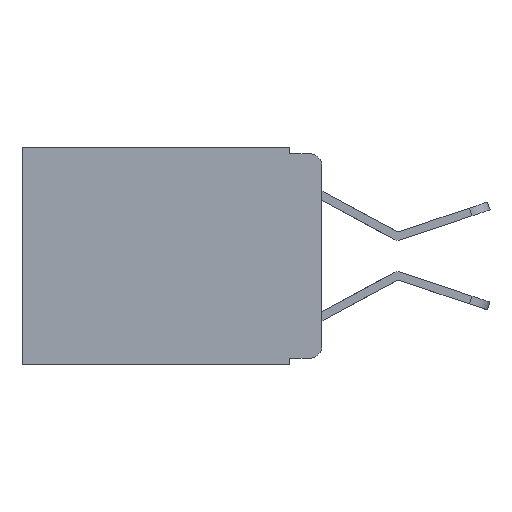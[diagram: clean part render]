
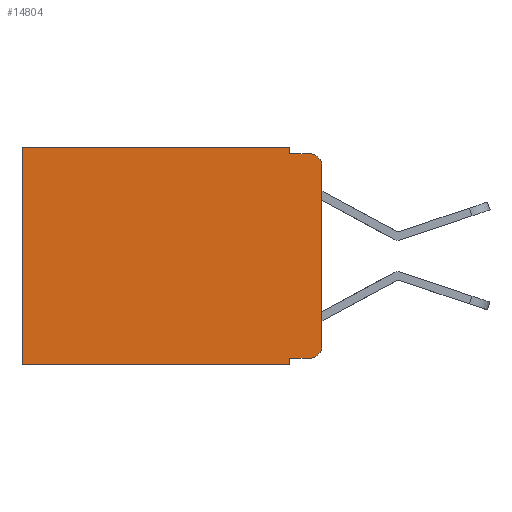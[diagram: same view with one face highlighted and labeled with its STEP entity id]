
A CAD part, left-side view. The second image highlights one B-rep face of the part: STEP entity #14804.
In plain terms, the highlighted planar face has unit normal (-1, 0, 0).
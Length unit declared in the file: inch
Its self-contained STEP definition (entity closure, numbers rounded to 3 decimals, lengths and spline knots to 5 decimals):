
#145 = DIRECTION ( 'NONE',  ( 0., 0., -1. ) ) ;
#515 = DIRECTION ( 'NONE',  ( 0., 0., -1. ) ) ;
#594 = CARTESIAN_POINT ( 'NONE',  ( 0.298, 0.02, -0.313 ) ) ;
#739 = ORIENTED_EDGE ( 'NONE', *, *, #18415, .T. ) ;
#830 = EDGE_CURVE ( 'NONE', #16625, #11333, #18608, .T. ) ;
#884 = FACE_OUTER_BOUND ( 'NONE', #12718, .T. ) ;
#1509 = CARTESIAN_POINT ( 'NONE',  ( 0.298, 0.051, 0. ) ) ;
#1631 = CARTESIAN_POINT ( 'NONE',  ( 0.298, 0., 0. ) ) ;
#1828 = VECTOR ( 'NONE', #9354, 39.37008 ) ;
#2371 = AXIS2_PLACEMENT_3D ( 'NONE', #19038, #20844, #145 ) ;
#2643 = VECTOR ( 'NONE', #6815, 39.37008 ) ;
#2956 = EDGE_CURVE ( 'NONE', #6185, #7506, #20419, .T. ) ;
#3319 = EDGE_CURVE ( 'NONE', #16625, #7506, #18123, .T. ) ;
#4558 = CARTESIAN_POINT ( 'NONE',  ( 0.298, 0., -0.03 ) ) ;
#5018 = CARTESIAN_POINT ( 'NONE',  ( 0.298, 0.051, -0.333 ) ) ;
#5165 = CARTESIAN_POINT ( 'NONE',  ( 0.298, 0.02, -0.01 ) ) ;
#5530 = ORIENTED_EDGE ( 'NONE', *, *, #18715, .T. ) ;
#5837 = DIRECTION ( 'NONE',  ( 1., 0., 0. ) ) ;
#6000 = DIRECTION ( 'NONE',  ( 0., -1., 0. ) ) ;
#6185 = VERTEX_POINT ( 'NONE', #9861 ) ;
#6274 = CARTESIAN_POINT ( 'NONE',  ( 0.298, 0.051, -0.343 ) ) ;
#6696 = CARTESIAN_POINT ( 'NONE',  ( 0.298, 0.051, 0. ) ) ;
#6815 = DIRECTION ( 'NONE',  ( 0., 1., 0. ) ) ;
#6839 = DIRECTION ( 'NONE',  ( 0., 0., -1. ) ) ;
#7383 = EDGE_CURVE ( 'NONE', #17297, #11333, #20947, .T. ) ;
#7386 = CARTESIAN_POINT ( 'NONE',  ( 0.298, 0., 0. ) ) ;
#7503 = DIRECTION ( 'NONE',  ( 0., 1., 0. ) ) ;
#7506 = VERTEX_POINT ( 'NONE', #13511 ) ;
#7632 = ORIENTED_EDGE ( 'NONE', *, *, #2956, .T. ) ;
#7813 = AXIS2_PLACEMENT_3D ( 'NONE', #15762, #5837, #12182 ) ;
#7970 = ORIENTED_EDGE ( 'NONE', *, *, #830, .T. ) ;
#8206 = ORIENTED_EDGE ( 'NONE', *, *, #13753, .F. ) ;
#8434 = CARTESIAN_POINT ( 'NONE',  ( 0.298, 0.051, -0.333 ) ) ;
#8742 = VECTOR ( 'NONE', #6839, 39.37008 ) ;
#9306 = LINE ( 'NONE', #8434, #14960 ) ;
#9354 = DIRECTION ( 'NONE',  ( 0., 0., -1. ) ) ;
#9387 = ORIENTED_EDGE ( 'NONE', *, *, #12958, .T. ) ;
#9861 = CARTESIAN_POINT ( 'NONE',  ( 0.298, 0.02, -0.333 ) ) ;
#9883 = CARTESIAN_POINT ( 'NONE',  ( 0.298, 0.473, 0. ) ) ;
#10683 = LINE ( 'NONE', #21407, #1828 ) ;
#11211 = ORIENTED_EDGE ( 'NONE', *, *, #3319, .F. ) ;
#11333 = VERTEX_POINT ( 'NONE', #5165 ) ;
#11559 = CARTESIAN_POINT ( 'NONE',  ( 0.298, 0.051, -0.01 ) ) ;
#11646 = AXIS2_PLACEMENT_3D ( 'NONE', #594, #19259, #515 ) ;
#11678 = CARTESIAN_POINT ( 'NONE',  ( 0.298, 0.051, -0.01 ) ) ;
#11801 = LINE ( 'NONE', #1631, #2643 ) ;
#12182 = DIRECTION ( 'NONE',  ( 0., 0., -1. ) ) ;
#12718 = EDGE_LOOP ( 'NONE', ( #11211, #7970, #20754, #8206, #739, #5530, #19837, #16620, #9387, #7632 ) ) ;
#12958 = EDGE_CURVE ( 'NONE', #20139, #6185, #9306, .T. ) ;
#13121 = DIRECTION ( 'NONE',  ( 0., -1., 0. ) ) ;
#13511 = CARTESIAN_POINT ( 'NONE',  ( 0.298, 0., -0.313 ) ) ;
#13753 = EDGE_CURVE ( 'NONE', #15507, #17297, #21929, .T. ) ;
#14804 = ADVANCED_FACE ( 'NONE', ( #884 ), #20848, .F. ) ;
#14960 = VECTOR ( 'NONE', #6000, 39.37008 ) ;
#15152 = EDGE_CURVE ( 'NONE', #20139, #17216, #17005, .T. ) ;
#15507 = VERTEX_POINT ( 'NONE', #6696 ) ;
#15529 = VECTOR ( 'NONE', #13121, 39.37008 ) ;
#15762 = CARTESIAN_POINT ( 'NONE',  ( 0.298, 0., 0. ) ) ;
#16180 = DIRECTION ( 'NONE',  ( 0., 0., -1. ) ) ;
#16318 = CARTESIAN_POINT ( 'NONE',  ( 0.298, 0.051, 0. ) ) ;
#16620 = ORIENTED_EDGE ( 'NONE', *, *, #15152, .F. ) ;
#16625 = VERTEX_POINT ( 'NONE', #4558 ) ;
#17005 = LINE ( 'NONE', #16318, #20525 ) ;
#17216 = VERTEX_POINT ( 'NONE', #6274 ) ;
#17297 = VERTEX_POINT ( 'NONE', #11678 ) ;
#17333 = CARTESIAN_POINT ( 'NONE',  ( 0.298, 0.473, -0.343 ) ) ;
#17797 = CARTESIAN_POINT ( 'NONE',  ( 0.298, 0., -0.343 ) ) ;
#18123 = LINE ( 'NONE', #7386, #20837 ) ;
#18415 = EDGE_CURVE ( 'NONE', #15507, #18767, #11801, .T. ) ;
#18608 = CIRCLE ( 'NONE', #2371, 0.02 ) ;
#18715 = EDGE_CURVE ( 'NONE', #18767, #20268, #10683, .T. ) ;
#18767 = VERTEX_POINT ( 'NONE', #9883 ) ;
#19030 = VECTOR ( 'NONE', #7503, 39.37008 ) ;
#19038 = CARTESIAN_POINT ( 'NONE',  ( 0.298, 0.02, -0.03 ) ) ;
#19259 = DIRECTION ( 'NONE',  ( -1., 0., 0. ) ) ;
#19662 = DIRECTION ( 'NONE',  ( 0., 0., -1. ) ) ;
#19833 = EDGE_CURVE ( 'NONE', #17216, #20268, #20669, .T. ) ;
#19837 = ORIENTED_EDGE ( 'NONE', *, *, #19833, .F. ) ;
#20139 = VERTEX_POINT ( 'NONE', #5018 ) ;
#20268 = VERTEX_POINT ( 'NONE', #17333 ) ;
#20419 = CIRCLE ( 'NONE', #11646, 0.02 ) ;
#20525 = VECTOR ( 'NONE', #16180, 39.37008 ) ;
#20669 = LINE ( 'NONE', #17797, #19030 ) ;
#20754 = ORIENTED_EDGE ( 'NONE', *, *, #7383, .F. ) ;
#20837 = VECTOR ( 'NONE', #19662, 39.37008 ) ;
#20844 = DIRECTION ( 'NONE',  ( -1., 0., 0. ) ) ;
#20848 = PLANE ( 'NONE',  #7813 ) ;
#20947 = LINE ( 'NONE', #11559, #15529 ) ;
#21407 = CARTESIAN_POINT ( 'NONE',  ( 0.298, 0.473, 0. ) ) ;
#21929 = LINE ( 'NONE', #1509, #8742 ) ;
